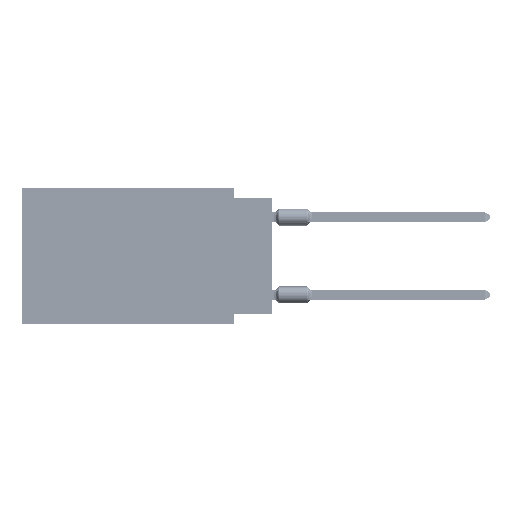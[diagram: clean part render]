
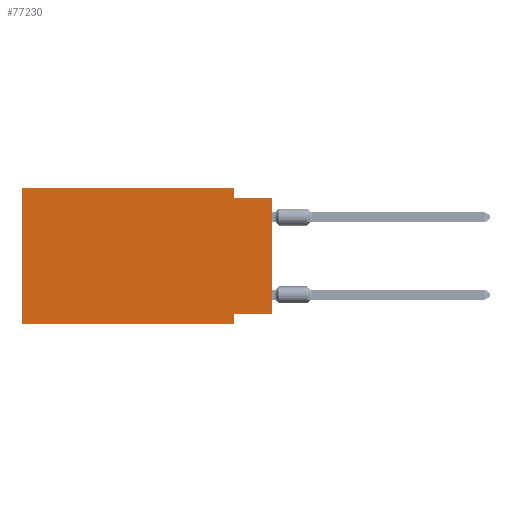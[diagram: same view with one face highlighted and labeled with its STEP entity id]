
A CAD part, left-side view. The second image highlights one B-rep face of the part: STEP entity #77230.
In plain terms, the highlighted planar face has unit normal (-1, 0, 0).
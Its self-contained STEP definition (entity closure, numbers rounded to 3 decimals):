
#1742 = EDGE_CURVE ( 'NONE', #31009, #32507, #18111, .T. ) ;
#2629 = EDGE_CURVE ( 'NONE', #15894, #4094, #39131, .T. ) ;
#3054 = EDGE_CURVE ( 'NONE', #4094, #91324, #58352, .T. ) ;
#4094 = VERTEX_POINT ( 'NONE', #85898 ) ;
#4683 = DIRECTION ( 'NONE',  ( 0., 1., 0. ) ) ;
#8311 = VECTOR ( 'NONE', #85883, 1000. ) ;
#9144 = DIRECTION ( 'NONE',  ( 0., -1., 0. ) ) ;
#9459 = EDGE_CURVE ( 'NONE', #63519, #40823, #24983, .T. ) ;
#11335 = DIRECTION ( 'NONE',  ( 0., 0., -1. ) ) ;
#12786 = CARTESIAN_POINT ( 'NONE',  ( 0., 2.54, 0. ) ) ;
#13225 = CARTESIAN_POINT ( 'NONE',  ( 0., 16.383, -8.89 ) ) ;
#15894 = VERTEX_POINT ( 'NONE', #13225 ) ;
#17162 = ORIENTED_EDGE ( 'NONE', *, *, #1742, .F. ) ;
#17821 = DIRECTION ( 'NONE',  ( 0., -1., 0. ) ) ;
#18111 = LINE ( 'NONE', #26773, #31266 ) ;
#19360 = DIRECTION ( 'NONE',  ( 1., 0., 0. ) ) ;
#21577 = EDGE_CURVE ( 'NONE', #63519, #31009, #49579, .T. ) ;
#21650 = CARTESIAN_POINT ( 'NONE',  ( 0., 16.383, 0. ) ) ;
#24983 = LINE ( 'NONE', #49083, #71154 ) ;
#25062 = CARTESIAN_POINT ( 'NONE',  ( 0., 16.383, -8.89 ) ) ;
#25195 = FACE_OUTER_BOUND ( 'NONE', #49207, .T. ) ;
#25411 = CARTESIAN_POINT ( 'NONE',  ( 0., 2.54, 0. ) ) ;
#26773 = CARTESIAN_POINT ( 'NONE',  ( 0., 2.54, -8.89 ) ) ;
#26922 = ORIENTED_EDGE ( 'NONE', *, *, #65093, .T. ) ;
#31009 = VERTEX_POINT ( 'NONE', #66168 ) ;
#31266 = VECTOR ( 'NONE', #11335, 1000. ) ;
#31373 = VECTOR ( 'NONE', #17821, 1000. ) ;
#32507 = VERTEX_POINT ( 'NONE', #70455 ) ;
#33687 = CARTESIAN_POINT ( 'NONE',  ( 0., 0., -8.255 ) ) ;
#37665 = LINE ( 'NONE', #67108, #93545 ) ;
#37879 = EDGE_CURVE ( 'NONE', #91324, #87575, #55816, .T. ) ;
#38657 = DIRECTION ( 'NONE',  ( 0., 0., 1. ) ) ;
#39131 = LINE ( 'NONE', #66667, #82343 ) ;
#40823 = VERTEX_POINT ( 'NONE', #84745 ) ;
#43686 = ORIENTED_EDGE ( 'NONE', *, *, #3054, .F. ) ;
#43986 = AXIS2_PLACEMENT_3D ( 'NONE', #56540, #19360, #84100 ) ;
#47198 = DIRECTION ( 'NONE',  ( 0., 0., 1. ) ) ;
#47416 = PLANE ( 'NONE',  #43986 ) ;
#49083 = CARTESIAN_POINT ( 'NONE',  ( 0., 0., 0. ) ) ;
#49207 = EDGE_LOOP ( 'NONE', ( #62870, #53070, #61648, #43686, #60331, #26922, #17162, #87618 ) ) ;
#49579 = LINE ( 'NONE', #33687, #81962 ) ;
#53070 = ORIENTED_EDGE ( 'NONE', *, *, #68907, .F. ) ;
#53190 = VECTOR ( 'NONE', #78467, 1000. ) ;
#55816 = LINE ( 'NONE', #12786, #53190 ) ;
#56416 = LINE ( 'NONE', #25062, #31373 ) ;
#56540 = CARTESIAN_POINT ( 'NONE',  ( 0., 16.383, 0. ) ) ;
#58352 = LINE ( 'NONE', #21650, #8311 ) ;
#60331 = ORIENTED_EDGE ( 'NONE', *, *, #2629, .F. ) ;
#61648 = ORIENTED_EDGE ( 'NONE', *, *, #37879, .F. ) ;
#62870 = ORIENTED_EDGE ( 'NONE', *, *, #9459, .T. ) ;
#63519 = VERTEX_POINT ( 'NONE', #63765 ) ;
#63765 = CARTESIAN_POINT ( 'NONE',  ( 0., 0., -8.255 ) ) ;
#65093 = EDGE_CURVE ( 'NONE', #15894, #32507, #56416, .T. ) ;
#66168 = CARTESIAN_POINT ( 'NONE',  ( 0., 2.54, -8.255 ) ) ;
#66667 = CARTESIAN_POINT ( 'NONE',  ( 0., 16.383, 0. ) ) ;
#67108 = CARTESIAN_POINT ( 'NONE',  ( 0., 0., -0.635 ) ) ;
#68907 = EDGE_CURVE ( 'NONE', #87575, #40823, #37665, .T. ) ;
#70455 = CARTESIAN_POINT ( 'NONE',  ( 0., 2.54, -8.89 ) ) ;
#71154 = VECTOR ( 'NONE', #47198, 1000. ) ;
#73190 = CARTESIAN_POINT ( 'NONE',  ( 0., 2.54, -0.635 ) ) ;
#77230 = ADVANCED_FACE ( 'NONE', ( #25195 ), #47416, .F. ) ;
#78467 = DIRECTION ( 'NONE',  ( 0., 0., -1. ) ) ;
#81962 = VECTOR ( 'NONE', #4683, 1000. ) ;
#82343 = VECTOR ( 'NONE', #38657, 1000. ) ;
#84100 = DIRECTION ( 'NONE',  ( 0., 0., -1. ) ) ;
#84745 = CARTESIAN_POINT ( 'NONE',  ( 0., 0., -0.635 ) ) ;
#85883 = DIRECTION ( 'NONE',  ( 0., -1., 0. ) ) ;
#85898 = CARTESIAN_POINT ( 'NONE',  ( 0., 16.383, 0. ) ) ;
#87575 = VERTEX_POINT ( 'NONE', #73190 ) ;
#87618 = ORIENTED_EDGE ( 'NONE', *, *, #21577, .F. ) ;
#91324 = VERTEX_POINT ( 'NONE', #25411 ) ;
#93545 = VECTOR ( 'NONE', #9144, 1000. ) ;
